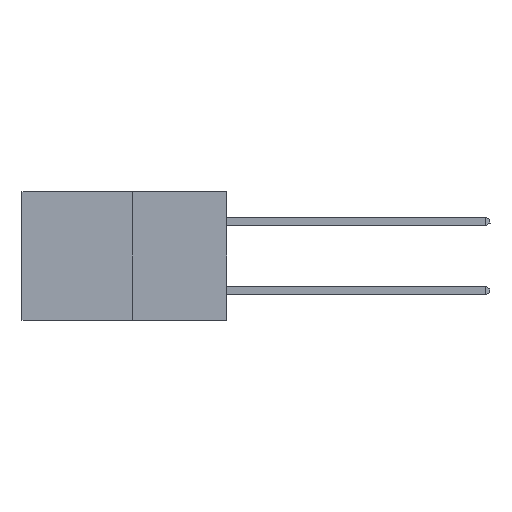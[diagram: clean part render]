
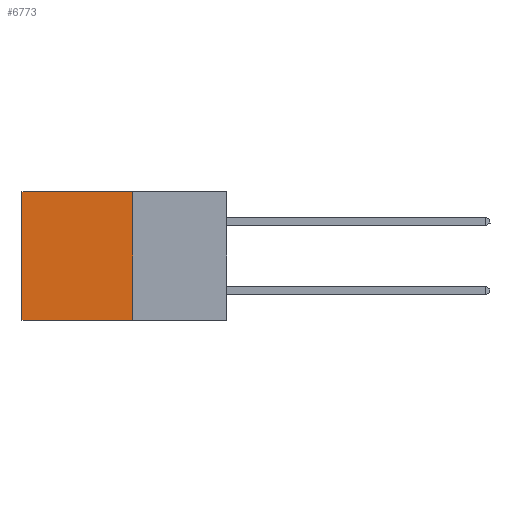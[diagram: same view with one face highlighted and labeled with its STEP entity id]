
A CAD part, left-side view. The second image highlights one B-rep face of the part: STEP entity #6773.
In plain terms, the highlighted planar face has unit normal (-1, 0, 0).
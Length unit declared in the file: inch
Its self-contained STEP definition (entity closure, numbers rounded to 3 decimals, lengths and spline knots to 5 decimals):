
#108 = VERTEX_POINT ( 'NONE', #4525 ) ;
#242 = AXIS2_PLACEMENT_3D ( 'NONE', #6233, #1501, #7031 ) ;
#270 = DIRECTION ( 'NONE',  ( 0., 0., -1. ) ) ;
#421 = DIRECTION ( 'NONE',  ( 0., 1., 0. ) ) ;
#525 = DIRECTION ( 'NONE',  ( 0., 1., 0. ) ) ;
#905 = FACE_OUTER_BOUND ( 'NONE', #6310, .T. ) ;
#1263 = CARTESIAN_POINT ( 'NONE',  ( 0.277, 0.27, -0.37 ) ) ;
#1428 = LINE ( 'NONE', #8132, #9759 ) ;
#1501 = DIRECTION ( 'NONE',  ( 1., 0., 0. ) ) ;
#1528 = LINE ( 'NONE', #9784, #5720 ) ;
#2588 = CARTESIAN_POINT ( 'NONE',  ( 0.277, 0.27, -0.37 ) ) ;
#2998 = ORIENTED_EDGE ( 'NONE', *, *, #4602, .T. ) ;
#3370 = VERTEX_POINT ( 'NONE', #9574 ) ;
#3461 = CARTESIAN_POINT ( 'NONE',  ( 0.277, 0.27, -0.37 ) ) ;
#4016 = VECTOR ( 'NONE', #7321, 39.37008 ) ;
#4525 = CARTESIAN_POINT ( 'NONE',  ( 0.277, 0.27, 0. ) ) ;
#4576 = EDGE_CURVE ( 'NONE', #108, #5335, #5864, .T. ) ;
#4602 = EDGE_CURVE ( 'NONE', #3370, #9795, #1428, .T. ) ;
#4609 = ORIENTED_EDGE ( 'NONE', *, *, #5478, .F. ) ;
#5090 = ORIENTED_EDGE ( 'NONE', *, *, #4576, .F. ) ;
#5335 = VERTEX_POINT ( 'NONE', #3461 ) ;
#5478 = EDGE_CURVE ( 'NONE', #5335, #9795, #6507, .T. ) ;
#5720 = VECTOR ( 'NONE', #421, 39.37008 ) ;
#5864 = LINE ( 'NONE', #2588, #4016 ) ;
#6233 = CARTESIAN_POINT ( 'NONE',  ( 0.277, 0.27, -0.37 ) ) ;
#6249 = VECTOR ( 'NONE', #525, 39.37008 ) ;
#6310 = EDGE_LOOP ( 'NONE', ( #2998, #4609, #5090, #7618 ) ) ;
#6478 = EDGE_CURVE ( 'NONE', #108, #3370, #1528, .T. ) ;
#6507 = LINE ( 'NONE', #1263, #6249 ) ;
#6773 = ADVANCED_FACE ( 'NONE', ( #905 ), #9332, .F. ) ;
#7031 = DIRECTION ( 'NONE',  ( 0., 0., -1. ) ) ;
#7321 = DIRECTION ( 'NONE',  ( 0., 0., -1. ) ) ;
#7618 = ORIENTED_EDGE ( 'NONE', *, *, #6478, .T. ) ;
#8132 = CARTESIAN_POINT ( 'NONE',  ( 0.277, 0.59, -0.37 ) ) ;
#8915 = CARTESIAN_POINT ( 'NONE',  ( 0.277, 0.59, -0.37 ) ) ;
#9332 = PLANE ( 'NONE',  #242 ) ;
#9574 = CARTESIAN_POINT ( 'NONE',  ( 0.277, 0.59, 0. ) ) ;
#9759 = VECTOR ( 'NONE', #270, 39.37008 ) ;
#9784 = CARTESIAN_POINT ( 'NONE',  ( 0.277, 0.27, 0. ) ) ;
#9795 = VERTEX_POINT ( 'NONE', #8915 ) ;
